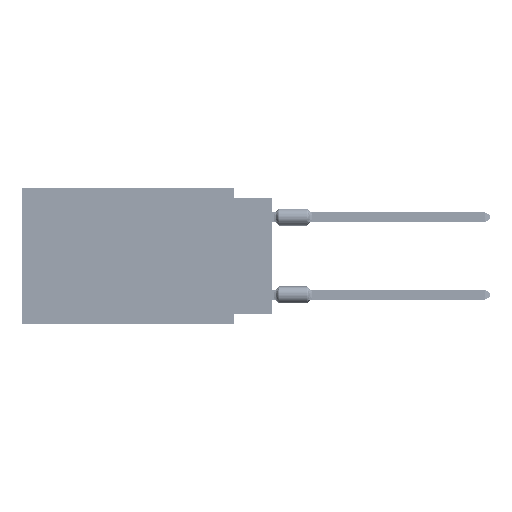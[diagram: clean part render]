
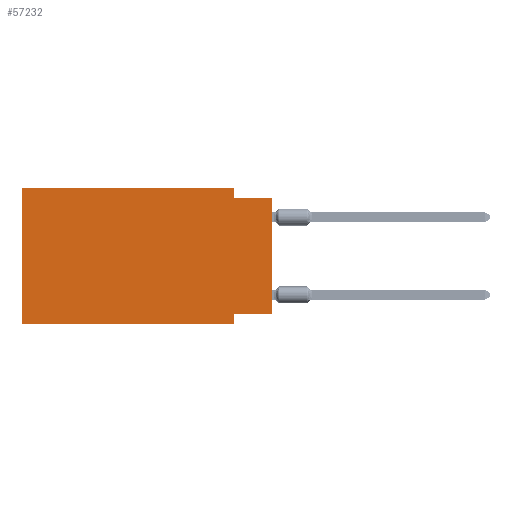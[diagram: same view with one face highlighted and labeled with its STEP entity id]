
A CAD part, left-side view. The second image highlights one B-rep face of the part: STEP entity #57232.
In plain terms, the highlighted planar face has unit normal (-1, 0, 0).
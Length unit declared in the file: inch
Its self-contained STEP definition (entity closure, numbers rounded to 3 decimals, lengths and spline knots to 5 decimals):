
#1519 = CARTESIAN_POINT ( 'NONE',  ( 0., 0.1, 0. ) ) ;
#3072 = VERTEX_POINT ( 'NONE', #69182 ) ;
#3883 = VECTOR ( 'NONE', #16454, 39.37008 ) ;
#5046 = DIRECTION ( 'NONE',  ( 0., -1., 0. ) ) ;
#6743 = CARTESIAN_POINT ( 'NONE',  ( 0., 0.645, -0.35 ) ) ;
#6881 = CARTESIAN_POINT ( 'NONE',  ( 0., 0.645, -0.35 ) ) ;
#6953 = ORIENTED_EDGE ( 'NONE', *, *, #16635, .F. ) ;
#9769 = LINE ( 'NONE', #28401, #3883 ) ;
#9938 = CARTESIAN_POINT ( 'NONE',  ( 0., 0., -0.025 ) ) ;
#10029 = DIRECTION ( 'NONE',  ( 0., 0., -1. ) ) ;
#13671 = ORIENTED_EDGE ( 'NONE', *, *, #16169, .F. ) ;
#14216 = FACE_OUTER_BOUND ( 'NONE', #45219, .T. ) ;
#15677 = VECTOR ( 'NONE', #34995, 39.37008 ) ;
#16142 = LINE ( 'NONE', #1519, #44960 ) ;
#16169 = EDGE_CURVE ( 'NONE', #44723, #54165, #32036, .T. ) ;
#16249 = LINE ( 'NONE', #9938, #73750 ) ;
#16454 = DIRECTION ( 'NONE',  ( 0., 0., 1. ) ) ;
#16608 = DIRECTION ( 'NONE',  ( 0., 0., 1. ) ) ;
#16635 = EDGE_CURVE ( 'NONE', #46565, #63810, #16249, .T. ) ;
#17450 = EDGE_CURVE ( 'NONE', #21297, #44723, #45112, .T. ) ;
#21297 = VERTEX_POINT ( 'NONE', #35541 ) ;
#21991 = EDGE_CURVE ( 'NONE', #27935, #54165, #51732, .T. ) ;
#22584 = LINE ( 'NONE', #62530, #25727 ) ;
#25727 = VECTOR ( 'NONE', #16608, 39.37008 ) ;
#26611 = VECTOR ( 'NONE', #52072, 39.37008 ) ;
#27935 = VERTEX_POINT ( 'NONE', #6743 ) ;
#28401 = CARTESIAN_POINT ( 'NONE',  ( 0., 0.645, 0. ) ) ;
#30860 = LINE ( 'NONE', #42067, #15677 ) ;
#31406 = CARTESIAN_POINT ( 'NONE',  ( 0., 0.645, 0. ) ) ;
#32036 = LINE ( 'NONE', #42495, #59514 ) ;
#34995 = DIRECTION ( 'NONE',  ( 0., -1., 0. ) ) ;
#35240 = EDGE_CURVE ( 'NONE', #41853, #46565, #16142, .T. ) ;
#35541 = CARTESIAN_POINT ( 'NONE',  ( 0., 0., -0.325 ) ) ;
#39511 = DIRECTION ( 'NONE',  ( 0., 1., 0. ) ) ;
#40215 = ORIENTED_EDGE ( 'NONE', *, *, #21991, .T. ) ;
#40700 = ORIENTED_EDGE ( 'NONE', *, *, #17450, .F. ) ;
#41106 = DIRECTION ( 'NONE',  ( 0., 0., -1. ) ) ;
#41853 = VERTEX_POINT ( 'NONE', #53892 ) ;
#42067 = CARTESIAN_POINT ( 'NONE',  ( 0., 0.645, 0. ) ) ;
#42495 = CARTESIAN_POINT ( 'NONE',  ( 0., 0.1, -0.35 ) ) ;
#44197 = EDGE_CURVE ( 'NONE', #3072, #41853, #30860, .T. ) ;
#44723 = VERTEX_POINT ( 'NONE', #58014 ) ;
#44960 = VECTOR ( 'NONE', #41106, 39.37008 ) ;
#45112 = LINE ( 'NONE', #56672, #71452 ) ;
#45219 = EDGE_LOOP ( 'NONE', ( #53024, #6953, #47347, #70441, #72933, #40215, #13671, #40700 ) ) ;
#45414 = EDGE_CURVE ( 'NONE', #27935, #3072, #9769, .T. ) ;
#46565 = VERTEX_POINT ( 'NONE', #68332 ) ;
#47347 = ORIENTED_EDGE ( 'NONE', *, *, #35240, .F. ) ;
#51732 = LINE ( 'NONE', #6881, #26611 ) ;
#52072 = DIRECTION ( 'NONE',  ( 0., -1., 0. ) ) ;
#53024 = ORIENTED_EDGE ( 'NONE', *, *, #56577, .T. ) ;
#53196 = CARTESIAN_POINT ( 'NONE',  ( 0., 0., -0.025 ) ) ;
#53412 = PLANE ( 'NONE',  #61573 ) ;
#53892 = CARTESIAN_POINT ( 'NONE',  ( 0., 0.1, 0. ) ) ;
#54165 = VERTEX_POINT ( 'NONE', #68007 ) ;
#56577 = EDGE_CURVE ( 'NONE', #21297, #63810, #22584, .T. ) ;
#56672 = CARTESIAN_POINT ( 'NONE',  ( 0., 0., -0.325 ) ) ;
#57232 = ADVANCED_FACE ( 'NONE', ( #14216 ), #53412, .F. ) ;
#58014 = CARTESIAN_POINT ( 'NONE',  ( 0., 0.1, -0.325 ) ) ;
#59514 = VECTOR ( 'NONE', #60791, 39.37008 ) ;
#60791 = DIRECTION ( 'NONE',  ( 0., 0., -1. ) ) ;
#61187 = DIRECTION ( 'NONE',  ( 1., 0., 0. ) ) ;
#61573 = AXIS2_PLACEMENT_3D ( 'NONE', #31406, #61187, #10029 ) ;
#62530 = CARTESIAN_POINT ( 'NONE',  ( 0., 0., 0. ) ) ;
#63810 = VERTEX_POINT ( 'NONE', #53196 ) ;
#68007 = CARTESIAN_POINT ( 'NONE',  ( 0., 0.1, -0.35 ) ) ;
#68332 = CARTESIAN_POINT ( 'NONE',  ( 0., 0.1, -0.025 ) ) ;
#69182 = CARTESIAN_POINT ( 'NONE',  ( 0., 0.645, 0. ) ) ;
#70441 = ORIENTED_EDGE ( 'NONE', *, *, #44197, .F. ) ;
#71452 = VECTOR ( 'NONE', #39511, 39.37008 ) ;
#72933 = ORIENTED_EDGE ( 'NONE', *, *, #45414, .F. ) ;
#73750 = VECTOR ( 'NONE', #5046, 39.37008 ) ;
